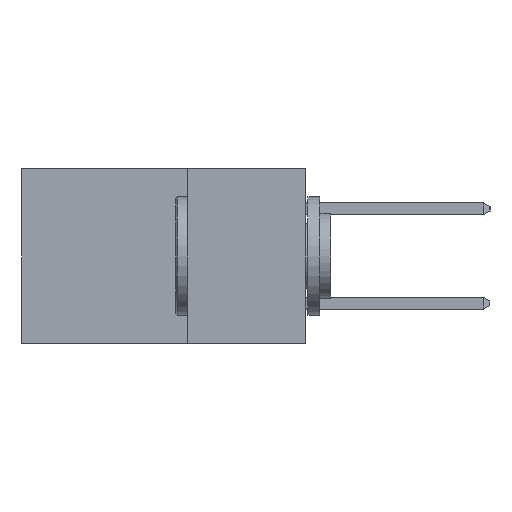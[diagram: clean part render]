
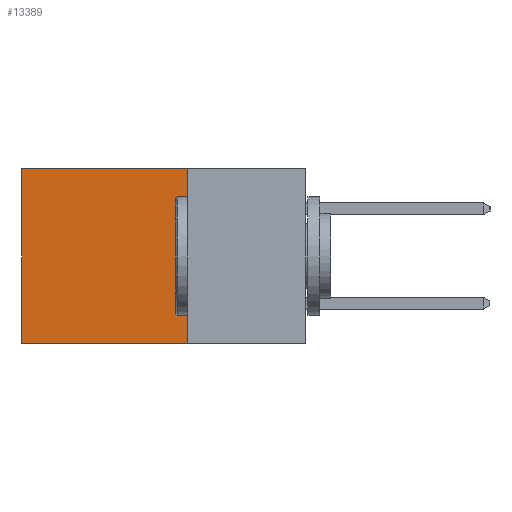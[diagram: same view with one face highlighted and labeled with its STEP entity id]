
A CAD part, left-side view. The second image highlights one B-rep face of the part: STEP entity #13389.
In plain terms, the highlighted planar face has unit normal (-1, 0, 0).
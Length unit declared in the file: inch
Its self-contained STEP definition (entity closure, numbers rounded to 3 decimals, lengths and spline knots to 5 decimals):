
#905 = EDGE_CURVE ( 'NONE', #3843, #17904, #1350, .T. ) ;
#1350 = LINE ( 'NONE', #19751, #10600 ) ;
#1412 = ORIENTED_EDGE ( 'NONE', *, *, #15275, .T. ) ;
#2335 = ORIENTED_EDGE ( 'NONE', *, *, #17690, .F. ) ;
#2451 = ORIENTED_EDGE ( 'NONE', *, *, #8879, .F. ) ;
#3058 = DIRECTION ( 'NONE',  ( 0., 0., -1. ) ) ;
#3349 = DIRECTION ( 'NONE',  ( 0., 0., -1. ) ) ;
#3437 = VECTOR ( 'NONE', #22960, 39.37008 ) ;
#3843 = VERTEX_POINT ( 'NONE', #20620 ) ;
#5715 = VECTOR ( 'NONE', #17901, 39.37008 ) ;
#7091 = CARTESIAN_POINT ( 'NONE',  ( 0.2615, 0.25, -0.37 ) ) ;
#8545 = ORIENTED_EDGE ( 'NONE', *, *, #905, .T. ) ;
#8879 = EDGE_CURVE ( 'NONE', #18511, #15610, #17946, .T. ) ;
#9166 = CARTESIAN_POINT ( 'NONE',  ( 0.2615, 0.25, 0. ) ) ;
#10180 = FACE_OUTER_BOUND ( 'NONE', #18286, .T. ) ;
#10600 = VECTOR ( 'NONE', #3349, 39.37008 ) ;
#11132 = CARTESIAN_POINT ( 'NONE',  ( 0.2615, 0.25, -0.37 ) ) ;
#11171 = CARTESIAN_POINT ( 'NONE',  ( 0.2615, 0.6, -0.37 ) ) ;
#12171 = CARTESIAN_POINT ( 'NONE',  ( 0.2615, 0.25, 0. ) ) ;
#12186 = PLANE ( 'NONE',  #15057 ) ;
#13389 = ADVANCED_FACE ( 'NONE', ( #10180 ), #12186, .F. ) ;
#13540 = LINE ( 'NONE', #12171, #23072 ) ;
#14009 = DIRECTION ( 'NONE',  ( 1., 0., 0. ) ) ;
#15057 = AXIS2_PLACEMENT_3D ( 'NONE', #19374, #14009, #3058 ) ;
#15275 = EDGE_CURVE ( 'NONE', #18511, #3843, #13540, .T. ) ;
#15610 = VERTEX_POINT ( 'NONE', #11132 ) ;
#15808 = DIRECTION ( 'NONE',  ( 0., 1., 0. ) ) ;
#17690 = EDGE_CURVE ( 'NONE', #15610, #17904, #20137, .T. ) ;
#17901 = DIRECTION ( 'NONE',  ( 0., 1., 0. ) ) ;
#17904 = VERTEX_POINT ( 'NONE', #11171 ) ;
#17946 = LINE ( 'NONE', #23324, #3437 ) ;
#18286 = EDGE_LOOP ( 'NONE', ( #8545, #2335, #2451, #1412 ) ) ;
#18511 = VERTEX_POINT ( 'NONE', #9166 ) ;
#19374 = CARTESIAN_POINT ( 'NONE',  ( 0.2615, 0.25, -0.37 ) ) ;
#19751 = CARTESIAN_POINT ( 'NONE',  ( 0.2615, 0.6, -0.37 ) ) ;
#20137 = LINE ( 'NONE', #7091, #5715 ) ;
#20620 = CARTESIAN_POINT ( 'NONE',  ( 0.2615, 0.6, 0. ) ) ;
#22960 = DIRECTION ( 'NONE',  ( 0., 0., -1. ) ) ;
#23072 = VECTOR ( 'NONE', #15808, 39.37008 ) ;
#23324 = CARTESIAN_POINT ( 'NONE',  ( 0.2615, 0.25, -0.37 ) ) ;
